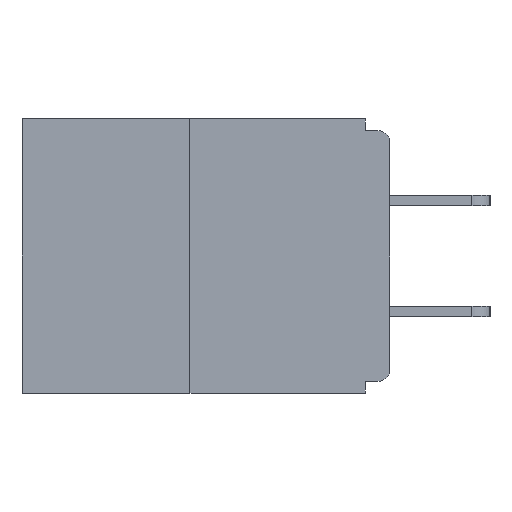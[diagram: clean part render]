
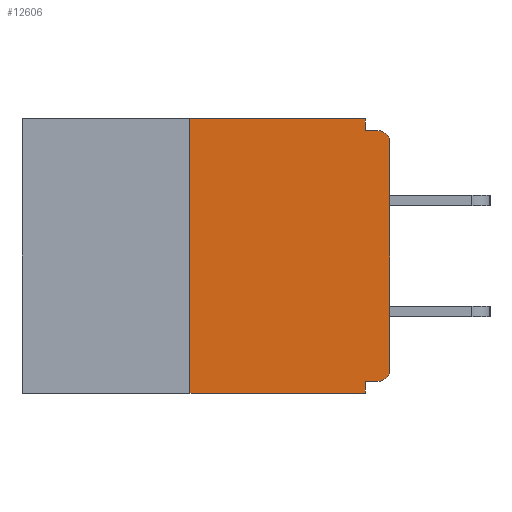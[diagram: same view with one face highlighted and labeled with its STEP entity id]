
A CAD part, left-side view. The second image highlights one B-rep face of the part: STEP entity #12606.
In plain terms, the highlighted planar face has unit normal (-1, 0, 0).
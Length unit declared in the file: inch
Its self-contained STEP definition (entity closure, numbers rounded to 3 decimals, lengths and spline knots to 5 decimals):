
#3 = CARTESIAN_POINT ( 'NONE',  ( 0., 0.25, -0.343 ) ) ;
#274 = CARTESIAN_POINT ( 'NONE',  ( 0., 0.25, 0. ) ) ;
#572 = DIRECTION ( 'NONE',  ( 0., 0., 1. ) ) ;
#594 = FACE_OUTER_BOUND ( 'NONE', #21045, .T. ) ;
#844 = ORIENTED_EDGE ( 'NONE', *, *, #5791, .F. ) ;
#907 = CARTESIAN_POINT ( 'NONE',  ( 0., 0.031, 0. ) ) ;
#1233 = VECTOR ( 'NONE', #572, 39.37008 ) ;
#1249 = CARTESIAN_POINT ( 'NONE',  ( 0., 0.46, 0. ) ) ;
#1444 = CARTESIAN_POINT ( 'NONE',  ( 0., 0.46, -0.343 ) ) ;
#2104 = CARTESIAN_POINT ( 'NONE',  ( 0., 0., -0.03 ) ) ;
#2105 = VECTOR ( 'NONE', #7470, 39.37008 ) ;
#2196 = DIRECTION ( 'NONE',  ( 0., 0., -1. ) ) ;
#2683 = VERTEX_POINT ( 'NONE', #274 ) ;
#2862 = LINE ( 'NONE', #1249, #12576 ) ;
#3397 = CARTESIAN_POINT ( 'NONE',  ( 0., 0.015, -0.03 ) ) ;
#3512 = DIRECTION ( 'NONE',  ( 0., -1., 0. ) ) ;
#3629 = CARTESIAN_POINT ( 'NONE',  ( 0., 0.015, -0.015 ) ) ;
#4036 = VECTOR ( 'NONE', #22186, 39.37008 ) ;
#4421 = VERTEX_POINT ( 'NONE', #3 ) ;
#4993 = ORIENTED_EDGE ( 'NONE', *, *, #17492, .F. ) ;
#5020 = CARTESIAN_POINT ( 'NONE',  ( 0., 0.015, -0.328 ) ) ;
#5097 = VERTEX_POINT ( 'NONE', #3629 ) ;
#5113 = VERTEX_POINT ( 'NONE', #12348 ) ;
#5406 = LINE ( 'NONE', #21089, #14712 ) ;
#5791 = EDGE_CURVE ( 'NONE', #12504, #18141, #16670, .T. ) ;
#7199 = CARTESIAN_POINT ( 'NONE',  ( 0., 0.25, 0. ) ) ;
#7223 = CARTESIAN_POINT ( 'NONE',  ( 0., 0.031, -0.328 ) ) ;
#7245 = DIRECTION ( 'NONE',  ( 0., 1., 0. ) ) ;
#7369 = EDGE_CURVE ( 'NONE', #4421, #18141, #19241, .T. ) ;
#7470 = DIRECTION ( 'NONE',  ( 0., 0., -1. ) ) ;
#7528 = ORIENTED_EDGE ( 'NONE', *, *, #21169, .T. ) ;
#7930 = CARTESIAN_POINT ( 'NONE',  ( 0., 0.031, -0.015 ) ) ;
#8338 = LINE ( 'NONE', #20553, #4036 ) ;
#9141 = VERTEX_POINT ( 'NONE', #2104 ) ;
#9172 = CARTESIAN_POINT ( 'NONE',  ( 0., 0.46, 0. ) ) ;
#10092 = ORIENTED_EDGE ( 'NONE', *, *, #14245, .F. ) ;
#10199 = ORIENTED_EDGE ( 'NONE', *, *, #10319, .F. ) ;
#10319 = EDGE_CURVE ( 'NONE', #16802, #5097, #13839, .T. ) ;
#10567 = VERTEX_POINT ( 'NONE', #5020 ) ;
#10801 = CARTESIAN_POINT ( 'NONE',  ( 0., 0.015, -0.313 ) ) ;
#10824 = LINE ( 'NONE', #12656, #20460 ) ;
#10915 = PLANE ( 'NONE',  #14865 ) ;
#11007 = DIRECTION ( 'NONE',  ( -1., 0., 0. ) ) ;
#11028 = EDGE_CURVE ( 'NONE', #5113, #9141, #8338, .T. ) ;
#11738 = AXIS2_PLACEMENT_3D ( 'NONE', #10801, #11007, #2196 ) ;
#12027 = EDGE_CURVE ( 'NONE', #10567, #12504, #5406, .T. ) ;
#12141 = CIRCLE ( 'NONE', #22458, 0.015 ) ;
#12348 = CARTESIAN_POINT ( 'NONE',  ( 0., 0., -0.313 ) ) ;
#12504 = VERTEX_POINT ( 'NONE', #7223 ) ;
#12576 = VECTOR ( 'NONE', #20193, 39.37008 ) ;
#12606 = ADVANCED_FACE ( 'NONE', ( #594 ), #10915, .F. ) ;
#12656 = CARTESIAN_POINT ( 'NONE',  ( 0., 0.031, 0. ) ) ;
#12975 = DIRECTION ( 'NONE',  ( 0., 0., -1. ) ) ;
#13592 = ORIENTED_EDGE ( 'NONE', *, *, #12027, .F. ) ;
#13616 = VECTOR ( 'NONE', #3512, 39.37008 ) ;
#13839 = LINE ( 'NONE', #19032, #14299 ) ;
#14245 = EDGE_CURVE ( 'NONE', #16425, #16802, #10824, .T. ) ;
#14299 = VECTOR ( 'NONE', #20650, 39.37008 ) ;
#14712 = VECTOR ( 'NONE', #7245, 39.37008 ) ;
#14865 = AXIS2_PLACEMENT_3D ( 'NONE', #9172, #17932, #12975 ) ;
#16425 = VERTEX_POINT ( 'NONE', #907 ) ;
#16670 = LINE ( 'NONE', #21629, #2105 ) ;
#16802 = VERTEX_POINT ( 'NONE', #7930 ) ;
#17492 = EDGE_CURVE ( 'NONE', #4421, #2683, #19744, .T. ) ;
#17853 = DIRECTION ( 'NONE',  ( 0., 0., -1. ) ) ;
#17932 = DIRECTION ( 'NONE',  ( 1., 0., 0. ) ) ;
#17996 = CIRCLE ( 'NONE', #11738, 0.015 ) ;
#18141 = VERTEX_POINT ( 'NONE', #22392 ) ;
#18176 = DIRECTION ( 'NONE',  ( 0., 0., -1. ) ) ;
#18194 = EDGE_CURVE ( 'NONE', #2683, #16425, #2862, .T. ) ;
#19032 = CARTESIAN_POINT ( 'NONE',  ( 0., 0., -0.015 ) ) ;
#19241 = LINE ( 'NONE', #1444, #13616 ) ;
#19744 = LINE ( 'NONE', #7199, #1233 ) ;
#20193 = DIRECTION ( 'NONE',  ( 0., -1., 0. ) ) ;
#20460 = VECTOR ( 'NONE', #18176, 39.37008 ) ;
#20553 = CARTESIAN_POINT ( 'NONE',  ( 0., 0., 0. ) ) ;
#20650 = DIRECTION ( 'NONE',  ( 0., -1., 0. ) ) ;
#21045 = EDGE_LOOP ( 'NONE', ( #22627, #4993, #22239, #844, #13592, #7528, #22630, #21127, #10199, #10092 ) ) ;
#21089 = CARTESIAN_POINT ( 'NONE',  ( 0., 0., -0.328 ) ) ;
#21127 = ORIENTED_EDGE ( 'NONE', *, *, #21856, .T. ) ;
#21169 = EDGE_CURVE ( 'NONE', #10567, #5113, #17996, .T. ) ;
#21629 = CARTESIAN_POINT ( 'NONE',  ( 0., 0.031, -0.343 ) ) ;
#21856 = EDGE_CURVE ( 'NONE', #9141, #5097, #12141, .T. ) ;
#22186 = DIRECTION ( 'NONE',  ( 0., 0., 1. ) ) ;
#22239 = ORIENTED_EDGE ( 'NONE', *, *, #7369, .T. ) ;
#22392 = CARTESIAN_POINT ( 'NONE',  ( 0., 0.031, -0.343 ) ) ;
#22458 = AXIS2_PLACEMENT_3D ( 'NONE', #3397, #22703, #17853 ) ;
#22627 = ORIENTED_EDGE ( 'NONE', *, *, #18194, .F. ) ;
#22630 = ORIENTED_EDGE ( 'NONE', *, *, #11028, .T. ) ;
#22703 = DIRECTION ( 'NONE',  ( -1., 0., 0. ) ) ;
